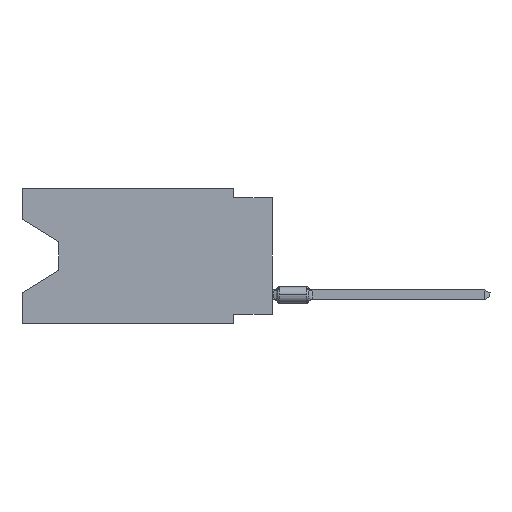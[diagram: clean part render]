
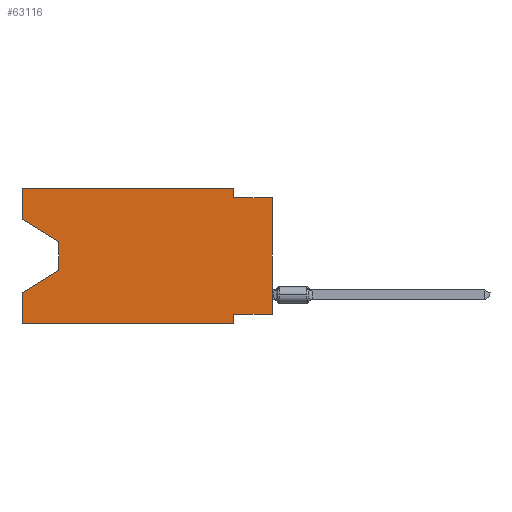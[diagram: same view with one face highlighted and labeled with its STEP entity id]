
A CAD part, left-side view. The second image highlights one B-rep face of the part: STEP entity #63116.
In plain terms, the highlighted planar face has unit normal (-1, 0, 0).
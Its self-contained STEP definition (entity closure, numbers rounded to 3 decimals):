
#10 = LINE ( 'NONE', #31589, #41955 ) ;
#13 = VECTOR ( 'NONE', #14195, 1000. ) ;
#1788 = EDGE_CURVE ( 'NONE', #63717, #60307, #5183, .T. ) ;
#2008 = CARTESIAN_POINT ( 'NONE',  ( 0., 2.54, -0.635 ) ) ;
#2190 = VERTEX_POINT ( 'NONE', #28004 ) ;
#2557 = CARTESIAN_POINT ( 'NONE',  ( 0., 2.54, 0. ) ) ;
#2893 = LINE ( 'NONE', #2557, #59441 ) ;
#3921 = CARTESIAN_POINT ( 'NONE',  ( 0., 2.54, -8.255 ) ) ;
#4645 = LINE ( 'NONE', #9779, #33650 ) ;
#4822 = DIRECTION ( 'NONE',  ( 0., 0., -1. ) ) ;
#5183 = LINE ( 'NONE', #26114, #16421 ) ;
#5497 = DIRECTION ( 'NONE',  ( 0., -0.855, -0.519 ) ) ;
#5767 = DIRECTION ( 'NONE',  ( 0., 0., -1. ) ) ;
#6119 = ORIENTED_EDGE ( 'NONE', *, *, #6840, .F. ) ;
#6840 = EDGE_CURVE ( 'NONE', #17078, #36812, #65794, .T. ) ;
#9779 = CARTESIAN_POINT ( 'NONE',  ( 0., 0., 0. ) ) ;
#10333 = EDGE_CURVE ( 'NONE', #21837, #27056, #67301, .T. ) ;
#12102 = CARTESIAN_POINT ( 'NONE',  ( 0., 13.97, -5.385 ) ) ;
#12471 = ORIENTED_EDGE ( 'NONE', *, *, #32969, .T. ) ;
#13834 = VECTOR ( 'NONE', #5767, 1000. ) ;
#14195 = DIRECTION ( 'NONE',  ( 0., 0., 1. ) ) ;
#15214 = CARTESIAN_POINT ( 'NONE',  ( 0., 16.383, 0. ) ) ;
#15545 = CARTESIAN_POINT ( 'NONE',  ( 0., 16.383, -8.89 ) ) ;
#16067 = FACE_OUTER_BOUND ( 'NONE', #33738, .T. ) ;
#16190 = CARTESIAN_POINT ( 'NONE',  ( 0., 16.383, -2.038 ) ) ;
#16421 = VECTOR ( 'NONE', #51512, 1000. ) ;
#16885 = VECTOR ( 'NONE', #55184, 1000. ) ;
#17078 = VERTEX_POINT ( 'NONE', #49705 ) ;
#17434 = VERTEX_POINT ( 'NONE', #24851 ) ;
#20015 = DIRECTION ( 'NONE',  ( 0., -1., 0. ) ) ;
#20291 = DIRECTION ( 'NONE',  ( 0., -1., 0. ) ) ;
#20364 = LINE ( 'NONE', #21640, #38631 ) ;
#20863 = PLANE ( 'NONE',  #54091 ) ;
#21640 = CARTESIAN_POINT ( 'NONE',  ( 0., 16.383, -8.89 ) ) ;
#21837 = VERTEX_POINT ( 'NONE', #2008 ) ;
#23826 = ORIENTED_EDGE ( 'NONE', *, *, #32765, .F. ) ;
#24404 = VECTOR ( 'NONE', #4822, 1000. ) ;
#24851 = CARTESIAN_POINT ( 'NONE',  ( 0., 16.383, -6.852 ) ) ;
#25832 = ORIENTED_EDGE ( 'NONE', *, *, #51046, .F. ) ;
#26114 = CARTESIAN_POINT ( 'NONE',  ( 0., 16.383, 0. ) ) ;
#26184 = ORIENTED_EDGE ( 'NONE', *, *, #36226, .F. ) ;
#27056 = VERTEX_POINT ( 'NONE', #28775 ) ;
#27628 = VECTOR ( 'NONE', #55114, 1000. ) ;
#27685 = CARTESIAN_POINT ( 'NONE',  ( 0., 13.97, -5.385 ) ) ;
#27977 = ORIENTED_EDGE ( 'NONE', *, *, #32814, .T. ) ;
#28004 = CARTESIAN_POINT ( 'NONE',  ( 0., 13.97, -3.505 ) ) ;
#28775 = CARTESIAN_POINT ( 'NONE',  ( 0., 0., -0.635 ) ) ;
#28976 = DIRECTION ( 'NONE',  ( 0., 0., -1. ) ) ;
#30245 = EDGE_CURVE ( 'NONE', #64436, #17434, #67034, .T. ) ;
#30368 = VERTEX_POINT ( 'NONE', #12102 ) ;
#31589 = CARTESIAN_POINT ( 'NONE',  ( 0., 16.383, -2.038 ) ) ;
#32765 = EDGE_CURVE ( 'NONE', #66116, #21837, #2893, .T. ) ;
#32814 = EDGE_CURVE ( 'NONE', #64436, #38359, #20364, .T. ) ;
#32969 = EDGE_CURVE ( 'NONE', #2190, #30368, #46457, .T. ) ;
#33094 = EDGE_CURVE ( 'NONE', #63717, #2190, #10, .T. ) ;
#33650 = VECTOR ( 'NONE', #67443, 1000. ) ;
#33738 = EDGE_LOOP ( 'NONE', ( #35431, #12471, #54633, #61965, #27977, #25832, #6119, #58595, #42989, #23826, #26184, #66396 ) ) ;
#35431 = ORIENTED_EDGE ( 'NONE', *, *, #33094, .T. ) ;
#36226 = EDGE_CURVE ( 'NONE', #60307, #66116, #52035, .T. ) ;
#36812 = VERTEX_POINT ( 'NONE', #3921 ) ;
#38359 = VERTEX_POINT ( 'NONE', #65303 ) ;
#38631 = VECTOR ( 'NONE', #20015, 1000. ) ;
#40719 = DIRECTION ( 'NONE',  ( 0., -1., 0. ) ) ;
#41955 = VECTOR ( 'NONE', #5497, 1000. ) ;
#42989 = ORIENTED_EDGE ( 'NONE', *, *, #10333, .F. ) ;
#43848 = CARTESIAN_POINT ( 'NONE',  ( 0., 2.54, -8.89 ) ) ;
#43937 = VECTOR ( 'NONE', #40719, 1000. ) ;
#44774 = EDGE_CURVE ( 'NONE', #30368, #17434, #64727, .T. ) ;
#45231 = CARTESIAN_POINT ( 'NONE',  ( 0., 0., -8.255 ) ) ;
#46457 = LINE ( 'NONE', #67369, #24404 ) ;
#46895 = CARTESIAN_POINT ( 'NONE',  ( 0., 16.383, 0. ) ) ;
#47313 = CARTESIAN_POINT ( 'NONE',  ( 0., 16.383, 0. ) ) ;
#49705 = CARTESIAN_POINT ( 'NONE',  ( 0., 0., -8.255 ) ) ;
#51046 = EDGE_CURVE ( 'NONE', #36812, #38359, #58273, .T. ) ;
#51512 = DIRECTION ( 'NONE',  ( 0., 0., 1. ) ) ;
#52035 = LINE ( 'NONE', #46895, #43937 ) ;
#52154 = CARTESIAN_POINT ( 'NONE',  ( 0., 16.383, 0. ) ) ;
#52526 = CARTESIAN_POINT ( 'NONE',  ( 0., 2.54, 0. ) ) ;
#54058 = EDGE_CURVE ( 'NONE', #17078, #27056, #4645, .T. ) ;
#54091 = AXIS2_PLACEMENT_3D ( 'NONE', #47313, #57920, #67542 ) ;
#54633 = ORIENTED_EDGE ( 'NONE', *, *, #44774, .T. ) ;
#55114 = DIRECTION ( 'NONE',  ( 0., 0.855, -0.519 ) ) ;
#55184 = DIRECTION ( 'NONE',  ( 0., 1., 0. ) ) ;
#55992 = CARTESIAN_POINT ( 'NONE',  ( 0., 0., -0.635 ) ) ;
#57920 = DIRECTION ( 'NONE',  ( 1., 0., 0. ) ) ;
#58273 = LINE ( 'NONE', #43848, #13834 ) ;
#58595 = ORIENTED_EDGE ( 'NONE', *, *, #54058, .T. ) ;
#59327 = VECTOR ( 'NONE', #20291, 1000. ) ;
#59441 = VECTOR ( 'NONE', #28976, 1000. ) ;
#60307 = VERTEX_POINT ( 'NONE', #52154 ) ;
#61965 = ORIENTED_EDGE ( 'NONE', *, *, #30245, .F. ) ;
#63116 = ADVANCED_FACE ( 'NONE', ( #16067 ), #20863, .F. ) ;
#63717 = VERTEX_POINT ( 'NONE', #16190 ) ;
#64436 = VERTEX_POINT ( 'NONE', #15545 ) ;
#64727 = LINE ( 'NONE', #27685, #27628 ) ;
#65303 = CARTESIAN_POINT ( 'NONE',  ( 0., 2.54, -8.89 ) ) ;
#65794 = LINE ( 'NONE', #45231, #16885 ) ;
#66116 = VERTEX_POINT ( 'NONE', #52526 ) ;
#66396 = ORIENTED_EDGE ( 'NONE', *, *, #1788, .F. ) ;
#67034 = LINE ( 'NONE', #15214, #13 ) ;
#67301 = LINE ( 'NONE', #55992, #59327 ) ;
#67369 = CARTESIAN_POINT ( 'NONE',  ( 0., 13.97, -3.505 ) ) ;
#67443 = DIRECTION ( 'NONE',  ( 0., 0., 1. ) ) ;
#67542 = DIRECTION ( 'NONE',  ( 0., 0., -1. ) ) ;
